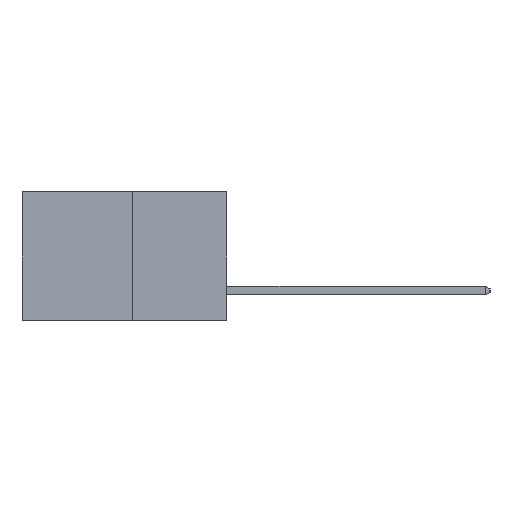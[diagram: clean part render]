
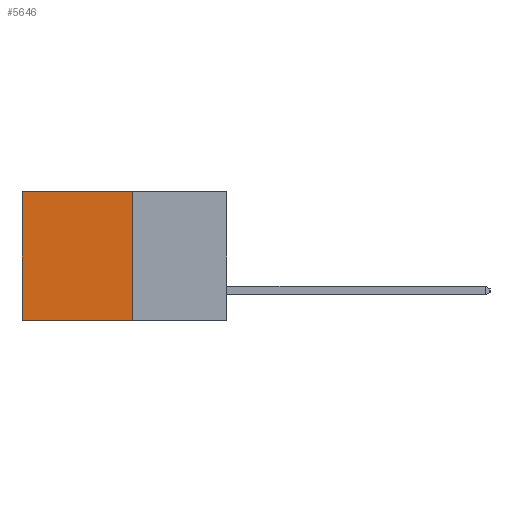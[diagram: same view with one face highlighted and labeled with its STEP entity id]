
A CAD part, left-side view. The second image highlights one B-rep face of the part: STEP entity #5646.
In plain terms, the highlighted planar face has unit normal (-1, 0, 0).
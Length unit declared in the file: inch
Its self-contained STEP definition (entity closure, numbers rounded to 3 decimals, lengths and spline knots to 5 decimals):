
#494 = VECTOR ( 'NONE', #9166, 39.37008 ) ;
#690 = CARTESIAN_POINT ( 'NONE',  ( 0.277, 0.59, -0.37 ) ) ;
#883 = DIRECTION ( 'NONE',  ( 0., 1., 0. ) ) ;
#982 = EDGE_LOOP ( 'NONE', ( #3195, #3848, #5661, #2047 ) ) ;
#1122 = VERTEX_POINT ( 'NONE', #6726 ) ;
#1178 = CARTESIAN_POINT ( 'NONE',  ( 0.277, 0.27, -0.37 ) ) ;
#1281 = DIRECTION ( 'NONE',  ( 0., 1., 0. ) ) ;
#1505 = CARTESIAN_POINT ( 'NONE',  ( 0.277, 0.27, 0. ) ) ;
#1593 = VERTEX_POINT ( 'NONE', #3561 ) ;
#2047 = ORIENTED_EDGE ( 'NONE', *, *, #4466, .T. ) ;
#2476 = VECTOR ( 'NONE', #4772, 39.37008 ) ;
#2571 = VECTOR ( 'NONE', #1281, 39.37008 ) ;
#2922 = FACE_OUTER_BOUND ( 'NONE', #982, .T. ) ;
#2943 = VERTEX_POINT ( 'NONE', #6101 ) ;
#2944 = LINE ( 'NONE', #9395, #494 ) ;
#3078 = VERTEX_POINT ( 'NONE', #3541 ) ;
#3195 = ORIENTED_EDGE ( 'NONE', *, *, #8874, .T. ) ;
#3541 = CARTESIAN_POINT ( 'NONE',  ( 0.277, 0.27, -0.37 ) ) ;
#3561 = CARTESIAN_POINT ( 'NONE',  ( 0.277, 0.59, 0. ) ) ;
#3848 = ORIENTED_EDGE ( 'NONE', *, *, #6433, .F. ) ;
#4466 = EDGE_CURVE ( 'NONE', #1122, #1593, #6798, .T. ) ;
#4689 = EDGE_CURVE ( 'NONE', #1122, #3078, #2944, .T. ) ;
#4772 = DIRECTION ( 'NONE',  ( 0., 0., -1. ) ) ;
#5485 = AXIS2_PLACEMENT_3D ( 'NONE', #7158, #7052, #7051 ) ;
#5578 = VECTOR ( 'NONE', #883, 39.37008 ) ;
#5646 = ADVANCED_FACE ( 'NONE', ( #2922 ), #7183, .F. ) ;
#5661 = ORIENTED_EDGE ( 'NONE', *, *, #4689, .F. ) ;
#6101 = CARTESIAN_POINT ( 'NONE',  ( 0.277, 0.59, -0.37 ) ) ;
#6433 = EDGE_CURVE ( 'NONE', #3078, #2943, #7588, .T. ) ;
#6726 = CARTESIAN_POINT ( 'NONE',  ( 0.277, 0.27, 0. ) ) ;
#6798 = LINE ( 'NONE', #1505, #2571 ) ;
#6949 = LINE ( 'NONE', #690, #2476 ) ;
#7051 = DIRECTION ( 'NONE',  ( 0., 0., -1. ) ) ;
#7052 = DIRECTION ( 'NONE',  ( 1., 0., 0. ) ) ;
#7158 = CARTESIAN_POINT ( 'NONE',  ( 0.277, 0.27, -0.37 ) ) ;
#7183 = PLANE ( 'NONE',  #5485 ) ;
#7588 = LINE ( 'NONE', #1178, #5578 ) ;
#8874 = EDGE_CURVE ( 'NONE', #1593, #2943, #6949, .T. ) ;
#9166 = DIRECTION ( 'NONE',  ( 0., 0., -1. ) ) ;
#9395 = CARTESIAN_POINT ( 'NONE',  ( 0.277, 0.27, -0.37 ) ) ;
